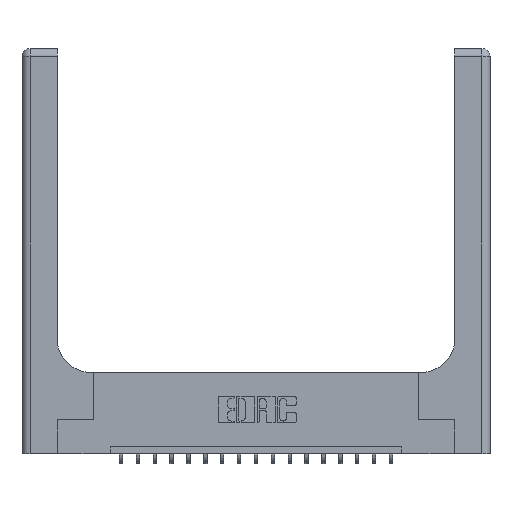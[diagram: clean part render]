
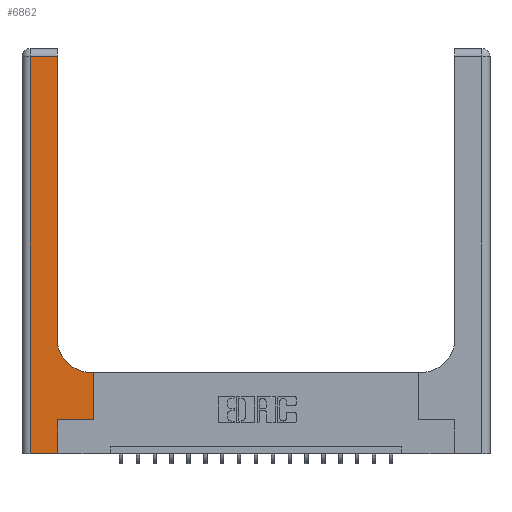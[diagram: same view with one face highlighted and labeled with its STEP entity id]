
A CAD part, top view. The second image highlights one B-rep face of the part: STEP entity #6862.
In plain terms, the highlighted planar face has unit normal (0, 0, 1).
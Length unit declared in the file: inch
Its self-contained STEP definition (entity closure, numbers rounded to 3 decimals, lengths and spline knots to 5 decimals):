
#24 = CARTESIAN_POINT ( 'NONE',  ( 0.51, 0.6, 0.37 ) ) ;
#792 = DIRECTION ( 'NONE',  ( 0., 0., -1. ) ) ;
#887 = CARTESIAN_POINT ( 'NONE',  ( 0.528, 0.25, 0.37 ) ) ;
#1228 = PLANE ( 'NONE',  #4300 ) ;
#1690 = CARTESIAN_POINT ( 'NONE',  ( 0.265, 0., 0.37 ) ) ;
#1789 = DIRECTION ( 'NONE',  ( 0., 1., 0. ) ) ;
#2275 = VERTEX_POINT ( 'NONE', #8171 ) ;
#2297 = CARTESIAN_POINT ( 'NONE',  ( 0.06, 3., 0.37 ) ) ;
#2416 = DIRECTION ( 'NONE',  ( -1., 0., 0. ) ) ;
#2573 = CARTESIAN_POINT ( 'NONE',  ( 0.51, 0.85, 0.37 ) ) ;
#2813 = CARTESIAN_POINT ( 'NONE',  ( 0., 3., 0.37 ) ) ;
#2906 = ORIENTED_EDGE ( 'NONE', *, *, #6389, .T. ) ;
#3207 = EDGE_CURVE ( 'NONE', #19053, #11176, #17245, .T. ) ;
#3256 = VECTOR ( 'NONE', #1789, 39.37008 ) ;
#3269 = CARTESIAN_POINT ( 'NONE',  ( 0.26, 3., 0.37 ) ) ;
#3527 = VERTEX_POINT ( 'NONE', #4310 ) ;
#3589 = CARTESIAN_POINT ( 'NONE',  ( 0.26, 2.94, 0.37 ) ) ;
#3835 = CARTESIAN_POINT ( 'NONE',  ( 0.265, 0.25, 0.37 ) ) ;
#3836 = VERTEX_POINT ( 'NONE', #3589 ) ;
#3892 = EDGE_CURVE ( 'NONE', #3527, #17136, #7727, .T. ) ;
#4183 = CARTESIAN_POINT ( 'NONE',  ( 0.528, 0.25, 0.37 ) ) ;
#4300 = AXIS2_PLACEMENT_3D ( 'NONE', #2813, #6083, #12136 ) ;
#4310 = CARTESIAN_POINT ( 'NONE',  ( 0.265, 0., 0.37 ) ) ;
#4838 = CARTESIAN_POINT ( 'NONE',  ( 0.06, 0., 0.37 ) ) ;
#5448 = DIRECTION ( 'NONE',  ( 1., 0., 0. ) ) ;
#5572 = EDGE_CURVE ( 'NONE', #3836, #9555, #9857, .T. ) ;
#5672 = DIRECTION ( 'NONE',  ( 0., -1., 0. ) ) ;
#6083 = DIRECTION ( 'NONE',  ( 0., 0., -1. ) ) ;
#6389 = EDGE_CURVE ( 'NONE', #17136, #11243, #14452, .T. ) ;
#6723 = AXIS2_PLACEMENT_3D ( 'NONE', #2573, #792, #5448 ) ;
#6862 = ADVANCED_FACE ( 'NONE', ( #11945 ), #1228, .F. ) ;
#7561 = EDGE_CURVE ( 'NONE', #11176, #3836, #16882, .T. ) ;
#7727 = LINE ( 'NONE', #1690, #3256 ) ;
#7826 = EDGE_CURVE ( 'NONE', #2275, #19053, #11694, .T. ) ;
#8171 = CARTESIAN_POINT ( 'NONE',  ( 0.528, 0.6, 0.37 ) ) ;
#8437 = ORIENTED_EDGE ( 'NONE', *, *, #17757, .T. ) ;
#8526 = ORIENTED_EDGE ( 'NONE', *, *, #7561, .T. ) ;
#8541 = EDGE_LOOP ( 'NONE', ( #8526, #13534, #9955, #8437, #9196, #2906, #17927, #10645, #17762 ) ) ;
#8938 = LINE ( 'NONE', #13806, #13279 ) ;
#9196 = ORIENTED_EDGE ( 'NONE', *, *, #3892, .T. ) ;
#9555 = VERTEX_POINT ( 'NONE', #18982 ) ;
#9857 = LINE ( 'NONE', #15915, #16947 ) ;
#9913 = CARTESIAN_POINT ( 'NONE',  ( 0.26, 0.85, 0.37 ) ) ;
#9955 = ORIENTED_EDGE ( 'NONE', *, *, #16479, .T. ) ;
#10630 = DIRECTION ( 'NONE',  ( 1., 0., 0. ) ) ;
#10645 = ORIENTED_EDGE ( 'NONE', *, *, #7826, .T. ) ;
#10948 = EDGE_CURVE ( 'NONE', #11243, #2275, #13516, .T. ) ;
#11176 = VERTEX_POINT ( 'NONE', #9913 ) ;
#11243 = VERTEX_POINT ( 'NONE', #887 ) ;
#11694 = LINE ( 'NONE', #17773, #12579 ) ;
#11945 = FACE_OUTER_BOUND ( 'NONE', #8541, .T. ) ;
#12136 = DIRECTION ( 'NONE',  ( -1., 0., 0. ) ) ;
#12579 = VECTOR ( 'NONE', #13389, 39.37008 ) ;
#13168 = DIRECTION ( 'NONE',  ( 1., 0., 0. ) ) ;
#13279 = VECTOR ( 'NONE', #10630, 39.37008 ) ;
#13389 = DIRECTION ( 'NONE',  ( -1., 0., 0. ) ) ;
#13516 = LINE ( 'NONE', #4183, #18527 ) ;
#13534 = ORIENTED_EDGE ( 'NONE', *, *, #5572, .T. ) ;
#13806 = CARTESIAN_POINT ( 'NONE',  ( 0., 0., 0.37 ) ) ;
#14452 = LINE ( 'NONE', #3835, #17621 ) ;
#14824 = CARTESIAN_POINT ( 'NONE',  ( 0.265, 0.25, 0.37 ) ) ;
#15008 = VERTEX_POINT ( 'NONE', #4838 ) ;
#15102 = VECTOR ( 'NONE', #15385, 39.37008 ) ;
#15385 = DIRECTION ( 'NONE',  ( 0., 1., 0. ) ) ;
#15915 = CARTESIAN_POINT ( 'NONE',  ( 0., 2.94, 0.37 ) ) ;
#16297 = DIRECTION ( 'NONE',  ( 0., 1., 0. ) ) ;
#16479 = EDGE_CURVE ( 'NONE', #9555, #15008, #19083, .T. ) ;
#16882 = LINE ( 'NONE', #3269, #15102 ) ;
#16947 = VECTOR ( 'NONE', #2416, 39.37008 ) ;
#17136 = VERTEX_POINT ( 'NONE', #14824 ) ;
#17245 = CIRCLE ( 'NONE', #6723, 0.25 ) ;
#17367 = VECTOR ( 'NONE', #5672, 39.37008 ) ;
#17621 = VECTOR ( 'NONE', #13168, 39.37008 ) ;
#17757 = EDGE_CURVE ( 'NONE', #15008, #3527, #8938, .T. ) ;
#17762 = ORIENTED_EDGE ( 'NONE', *, *, #3207, .T. ) ;
#17773 = CARTESIAN_POINT ( 'NONE',  ( 0.26, 0.6, 0.37 ) ) ;
#17927 = ORIENTED_EDGE ( 'NONE', *, *, #10948, .T. ) ;
#18527 = VECTOR ( 'NONE', #16297, 39.37008 ) ;
#18982 = CARTESIAN_POINT ( 'NONE',  ( 0.06, 2.94, 0.37 ) ) ;
#19053 = VERTEX_POINT ( 'NONE', #24 ) ;
#19083 = LINE ( 'NONE', #2297, #17367 ) ;
